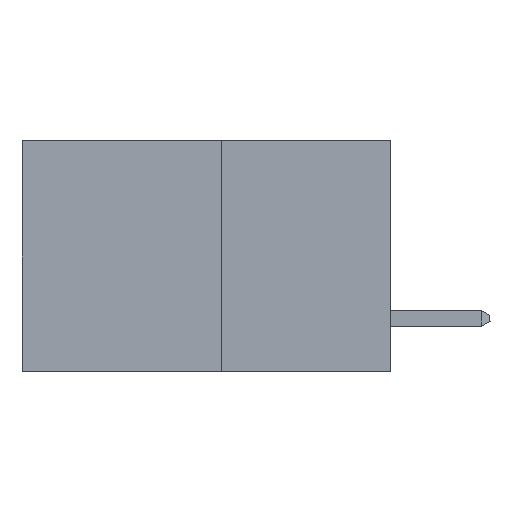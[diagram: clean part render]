
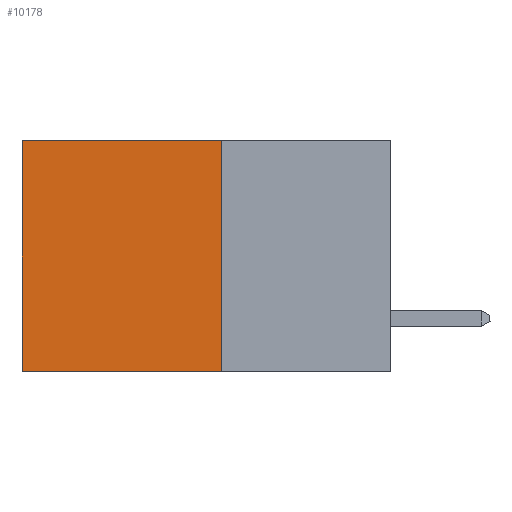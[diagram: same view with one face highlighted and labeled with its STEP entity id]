
A CAD part, left-side view. The second image highlights one B-rep face of the part: STEP entity #10178.
In plain terms, the highlighted planar face has unit normal (-1, 0, 0).
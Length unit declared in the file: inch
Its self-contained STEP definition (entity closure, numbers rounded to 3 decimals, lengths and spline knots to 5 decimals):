
#256 = FACE_OUTER_BOUND ( 'NONE', #10480, .T. ) ;
#580 = EDGE_CURVE ( 'NONE', #16027, #9130, #10478, .T. ) ;
#1473 = CARTESIAN_POINT ( 'NONE',  ( 0.277, 0.27, -0.37 ) ) ;
#1774 = VERTEX_POINT ( 'NONE', #16441 ) ;
#2000 = VERTEX_POINT ( 'NONE', #13138 ) ;
#2595 = DIRECTION ( 'NONE',  ( 0., 0., -1. ) ) ;
#2802 = DIRECTION ( 'NONE',  ( 0., 1., 0. ) ) ;
#3552 = EDGE_CURVE ( 'NONE', #2000, #1774, #8314, .T. ) ;
#4360 = VECTOR ( 'NONE', #15777, 39.37008 ) ;
#5611 = VECTOR ( 'NONE', #14095, 39.37008 ) ;
#6105 = LINE ( 'NONE', #15752, #8410 ) ;
#7165 = VECTOR ( 'NONE', #2802, 39.37008 ) ;
#7254 = EDGE_CURVE ( 'NONE', #2000, #16027, #6105, .T. ) ;
#7577 = LINE ( 'NONE', #1473, #7165 ) ;
#7788 = PLANE ( 'NONE',  #11982 ) ;
#8314 = LINE ( 'NONE', #10867, #4360 ) ;
#8410 = VECTOR ( 'NONE', #9526, 39.37008 ) ;
#9090 = CARTESIAN_POINT ( 'NONE',  ( 0.277, 0.27, -0.37 ) ) ;
#9130 = VERTEX_POINT ( 'NONE', #14505 ) ;
#9526 = DIRECTION ( 'NONE',  ( 0., 1., 0. ) ) ;
#10178 = ADVANCED_FACE ( 'NONE', ( #256 ), #7788, .F. ) ;
#10404 = DIRECTION ( 'NONE',  ( 1., 0., 0. ) ) ;
#10461 = ORIENTED_EDGE ( 'NONE', *, *, #3552, .F. ) ;
#10478 = LINE ( 'NONE', #11040, #5611 ) ;
#10480 = EDGE_LOOP ( 'NONE', ( #13021, #16267, #10461, #13817 ) ) ;
#10867 = CARTESIAN_POINT ( 'NONE',  ( 0.277, 0.27, -0.37 ) ) ;
#11040 = CARTESIAN_POINT ( 'NONE',  ( 0.277, 0.59, -0.37 ) ) ;
#11982 = AXIS2_PLACEMENT_3D ( 'NONE', #9090, #10404, #2595 ) ;
#12863 = EDGE_CURVE ( 'NONE', #1774, #9130, #7577, .T. ) ;
#13021 = ORIENTED_EDGE ( 'NONE', *, *, #580, .T. ) ;
#13138 = CARTESIAN_POINT ( 'NONE',  ( 0.277, 0.27, 0. ) ) ;
#13342 = CARTESIAN_POINT ( 'NONE',  ( 0.277, 0.59, 0. ) ) ;
#13817 = ORIENTED_EDGE ( 'NONE', *, *, #7254, .T. ) ;
#14095 = DIRECTION ( 'NONE',  ( 0., 0., -1. ) ) ;
#14505 = CARTESIAN_POINT ( 'NONE',  ( 0.277, 0.59, -0.37 ) ) ;
#15752 = CARTESIAN_POINT ( 'NONE',  ( 0.277, 0.27, 0. ) ) ;
#15777 = DIRECTION ( 'NONE',  ( 0., 0., -1. ) ) ;
#16027 = VERTEX_POINT ( 'NONE', #13342 ) ;
#16267 = ORIENTED_EDGE ( 'NONE', *, *, #12863, .F. ) ;
#16441 = CARTESIAN_POINT ( 'NONE',  ( 0.277, 0.27, -0.37 ) ) ;
